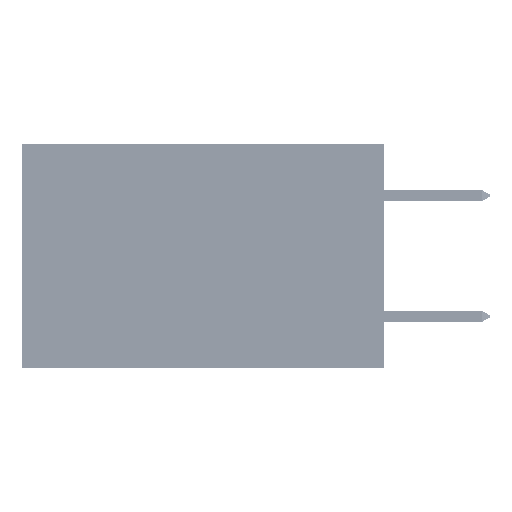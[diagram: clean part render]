
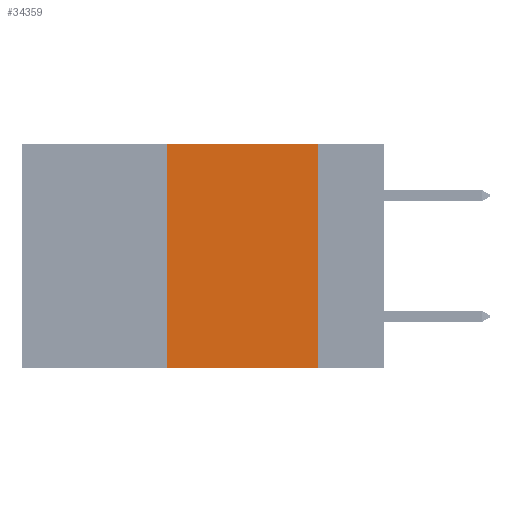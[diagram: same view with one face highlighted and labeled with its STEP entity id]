
A CAD part, left-side view. The second image highlights one B-rep face of the part: STEP entity #34359.
In plain terms, the highlighted planar face has unit normal (-1, 0, 0).
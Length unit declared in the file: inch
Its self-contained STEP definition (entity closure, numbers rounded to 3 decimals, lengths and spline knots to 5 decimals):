
#262 = CARTESIAN_POINT ( 'NONE',  ( 0., 0.11, 0. ) ) ;
#1043 = ORIENTED_EDGE ( 'NONE', *, *, #21389, .T. ) ;
#1284 = LINE ( 'NONE', #34341, #19705 ) ;
#1609 = EDGE_CURVE ( 'NONE', #45586, #4362, #26020, .T. ) ;
#2053 = EDGE_CURVE ( 'NONE', #4362, #25423, #1284, .T. ) ;
#3055 = AXIS2_PLACEMENT_3D ( 'NONE', #5685, #5542, #31215 ) ;
#3218 = CARTESIAN_POINT ( 'NONE',  ( 0., 0.36, 0. ) ) ;
#4362 = VERTEX_POINT ( 'NONE', #29141 ) ;
#5542 = DIRECTION ( 'NONE',  ( 1., 0., 0. ) ) ;
#5685 = CARTESIAN_POINT ( 'NONE',  ( 0., 0.6, 0. ) ) ;
#5723 = VERTEX_POINT ( 'NONE', #29647 ) ;
#7369 = DIRECTION ( 'NONE',  ( 0., 0., 1. ) ) ;
#9590 = EDGE_LOOP ( 'NONE', ( #31301, #41148, #16088, #1043 ) ) ;
#14213 = DIRECTION ( 'NONE',  ( 0., -1., 0. ) ) ;
#15899 = CARTESIAN_POINT ( 'NONE',  ( 0., 0.36, -0.37 ) ) ;
#16088 = ORIENTED_EDGE ( 'NONE', *, *, #1609, .F. ) ;
#17625 = FACE_OUTER_BOUND ( 'NONE', #9590, .T. ) ;
#18768 = DIRECTION ( 'NONE',  ( 0., 0., -1. ) ) ;
#19705 = VECTOR ( 'NONE', #26509, 39.37008 ) ;
#21389 = EDGE_CURVE ( 'NONE', #45586, #5723, #37834, .T. ) ;
#24829 = CARTESIAN_POINT ( 'NONE',  ( 0., 0.6, -0.37 ) ) ;
#25423 = VERTEX_POINT ( 'NONE', #40226 ) ;
#26020 = LINE ( 'NONE', #3218, #34069 ) ;
#26509 = DIRECTION ( 'NONE',  ( 0., -1., 0. ) ) ;
#29141 = CARTESIAN_POINT ( 'NONE',  ( 0., 0.36, 0. ) ) ;
#29647 = CARTESIAN_POINT ( 'NONE',  ( 0., 0.11, -0.37 ) ) ;
#31215 = DIRECTION ( 'NONE',  ( 0., 0., -1. ) ) ;
#31301 = ORIENTED_EDGE ( 'NONE', *, *, #35237, .F. ) ;
#34069 = VECTOR ( 'NONE', #7369, 39.37008 ) ;
#34341 = CARTESIAN_POINT ( 'NONE',  ( 0., 0.6, 0. ) ) ;
#34359 = ADVANCED_FACE ( 'NONE', ( #17625 ), #34734, .F. ) ;
#34734 = PLANE ( 'NONE',  #3055 ) ;
#35237 = EDGE_CURVE ( 'NONE', #25423, #5723, #37221, .T. ) ;
#37221 = LINE ( 'NONE', #262, #40676 ) ;
#37834 = LINE ( 'NONE', #24829, #41880 ) ;
#40226 = CARTESIAN_POINT ( 'NONE',  ( 0., 0.11, 0. ) ) ;
#40676 = VECTOR ( 'NONE', #18768, 39.37008 ) ;
#41148 = ORIENTED_EDGE ( 'NONE', *, *, #2053, .F. ) ;
#41880 = VECTOR ( 'NONE', #14213, 39.37008 ) ;
#45586 = VERTEX_POINT ( 'NONE', #15899 ) ;
